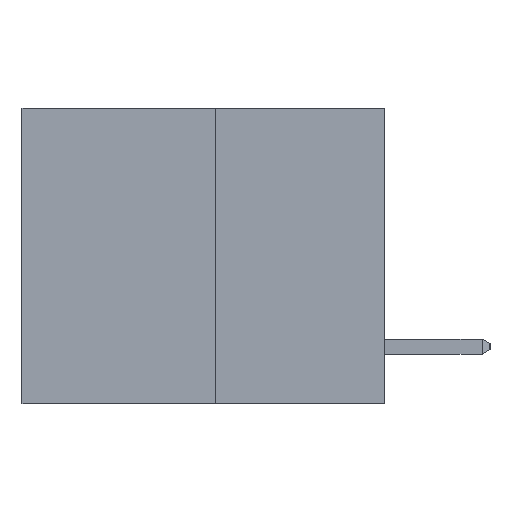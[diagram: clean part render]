
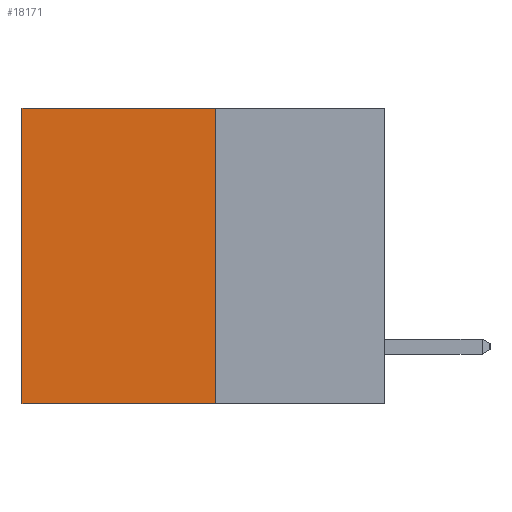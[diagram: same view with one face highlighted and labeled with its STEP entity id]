
A CAD part, left-side view. The second image highlights one B-rep face of the part: STEP entity #18171.
In plain terms, the highlighted planar face has unit normal (-1, 0, 0).
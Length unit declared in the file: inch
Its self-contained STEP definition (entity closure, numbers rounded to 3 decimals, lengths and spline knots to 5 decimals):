
#536 = FACE_OUTER_BOUND ( 'NONE', #17532, .T. ) ;
#1045 = CARTESIAN_POINT ( 'NONE',  ( 0.3165, 0.28, -0.49 ) ) ;
#1164 = ORIENTED_EDGE ( 'NONE', *, *, #4729, .T. ) ;
#3947 = ORIENTED_EDGE ( 'NONE', *, *, #11955, .F. ) ;
#4729 = EDGE_CURVE ( 'NONE', #21033, #8987, #13211, .T. ) ;
#5535 = DIRECTION ( 'NONE',  ( 0., 1., 0. ) ) ;
#6394 = DIRECTION ( 'NONE',  ( 0., 1., 0. ) ) ;
#6415 = VECTOR ( 'NONE', #6394, 39.37008 ) ;
#6936 = LINE ( 'NONE', #14764, #6415 ) ;
#7661 = DIRECTION ( 'NONE',  ( 1., 0., 0. ) ) ;
#7843 = LINE ( 'NONE', #21733, #17890 ) ;
#8082 = VERTEX_POINT ( 'NONE', #20681 ) ;
#8290 = EDGE_CURVE ( 'NONE', #8987, #17243, #17855, .T. ) ;
#8987 = VERTEX_POINT ( 'NONE', #12080 ) ;
#10261 = CARTESIAN_POINT ( 'NONE',  ( 0.3165, 0.28, 0. ) ) ;
#11955 = EDGE_CURVE ( 'NONE', #8082, #17243, #6936, .T. ) ;
#12080 = CARTESIAN_POINT ( 'NONE',  ( 0.3165, 0.6, 0. ) ) ;
#12746 = AXIS2_PLACEMENT_3D ( 'NONE', #1045, #7661, #15907 ) ;
#13211 = LINE ( 'NONE', #18771, #20634 ) ;
#13603 = CARTESIAN_POINT ( 'NONE',  ( 0.3165, 0.6, -0.49 ) ) ;
#13747 = DIRECTION ( 'NONE',  ( 0., 0., -1. ) ) ;
#13808 = EDGE_CURVE ( 'NONE', #21033, #8082, #7843, .T. ) ;
#14130 = VECTOR ( 'NONE', #13747, 39.37008 ) ;
#14215 = PLANE ( 'NONE',  #12746 ) ;
#14764 = CARTESIAN_POINT ( 'NONE',  ( 0.3165, 0.28, -0.49 ) ) ;
#14981 = DIRECTION ( 'NONE',  ( 0., 0., -1. ) ) ;
#15440 = ORIENTED_EDGE ( 'NONE', *, *, #13808, .F. ) ;
#15907 = DIRECTION ( 'NONE',  ( 0., 0., -1. ) ) ;
#16179 = ORIENTED_EDGE ( 'NONE', *, *, #8290, .T. ) ;
#17243 = VERTEX_POINT ( 'NONE', #13603 ) ;
#17532 = EDGE_LOOP ( 'NONE', ( #16179, #3947, #15440, #1164 ) ) ;
#17855 = LINE ( 'NONE', #18424, #14130 ) ;
#17890 = VECTOR ( 'NONE', #14981, 39.37008 ) ;
#18171 = ADVANCED_FACE ( 'NONE', ( #536 ), #14215, .F. ) ;
#18424 = CARTESIAN_POINT ( 'NONE',  ( 0.3165, 0.6, -0.49 ) ) ;
#18771 = CARTESIAN_POINT ( 'NONE',  ( 0.3165, 0.28, 0. ) ) ;
#20634 = VECTOR ( 'NONE', #5535, 39.37008 ) ;
#20681 = CARTESIAN_POINT ( 'NONE',  ( 0.3165, 0.28, -0.49 ) ) ;
#21033 = VERTEX_POINT ( 'NONE', #10261 ) ;
#21733 = CARTESIAN_POINT ( 'NONE',  ( 0.3165, 0.28, -0.49 ) ) ;
